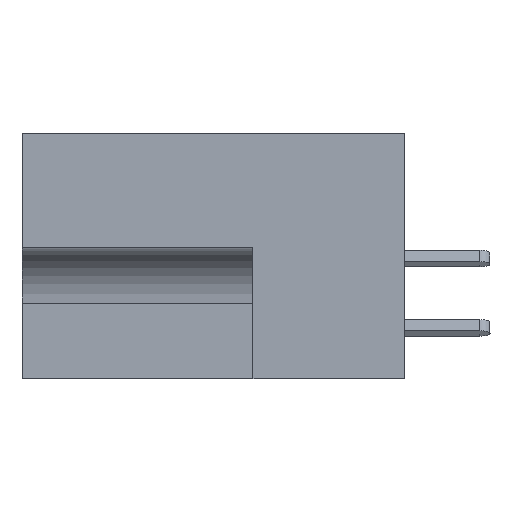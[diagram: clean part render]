
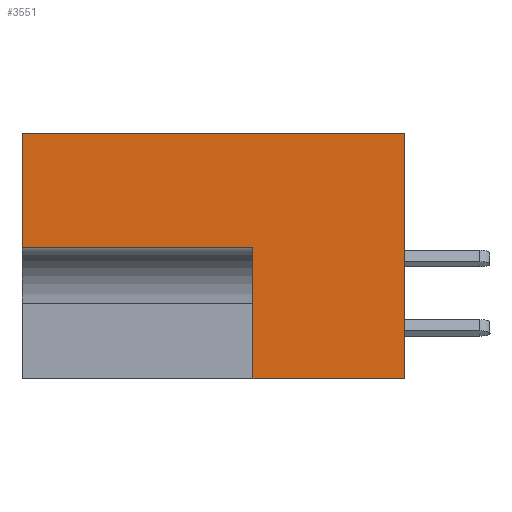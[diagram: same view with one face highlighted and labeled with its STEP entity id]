
A CAD part, left-side view. The second image highlights one B-rep face of the part: STEP entity #3551.
In plain terms, the highlighted planar face has unit normal (-1, 0, 0).
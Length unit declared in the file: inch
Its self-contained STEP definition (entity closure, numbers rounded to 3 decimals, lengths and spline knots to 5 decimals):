
#204 = VERTEX_POINT ( 'NONE', #14856 ) ;
#219 = LINE ( 'NONE', #20313, #17202 ) ;
#373 = DIRECTION ( 'NONE',  ( 0., -1., 0. ) ) ;
#418 = LINE ( 'NONE', #9601, #9098 ) ;
#633 = DIRECTION ( 'NONE',  ( 0., 0., 1. ) ) ;
#1474 = EDGE_CURVE ( 'NONE', #8236, #1812, #13132, .T. ) ;
#1812 = VERTEX_POINT ( 'NONE', #20797 ) ;
#2389 = VECTOR ( 'NONE', #18002, 39.37008 ) ;
#2929 = CARTESIAN_POINT ( 'NONE',  ( 0., 0.328, -0.531 ) ) ;
#3551 = ADVANCED_FACE ( 'NONE', ( #16858 ), #7115, .F. ) ;
#4475 = LINE ( 'NONE', #2929, #2389 ) ;
#4581 = EDGE_CURVE ( 'NONE', #20602, #10920, #5206, .T. ) ;
#5206 = LINE ( 'NONE', #12633, #23700 ) ;
#7115 = PLANE ( 'NONE',  #20609 ) ;
#7203 = CARTESIAN_POINT ( 'NONE',  ( 0., 0.453, 0. ) ) ;
#7913 = CARTESIAN_POINT ( 'NONE',  ( 0., 0.828, 0. ) ) ;
#8236 = VERTEX_POINT ( 'NONE', #7913 ) ;
#8436 = CARTESIAN_POINT ( 'NONE',  ( 0., 0.328, -0.531 ) ) ;
#8957 = DIRECTION ( 'NONE',  ( 0., -1., 0. ) ) ;
#9098 = VECTOR ( 'NONE', #22949, 39.37008 ) ;
#9601 = CARTESIAN_POINT ( 'NONE',  ( 0., 0.328, -0.248 ) ) ;
#9984 = ORIENTED_EDGE ( 'NONE', *, *, #19945, .F. ) ;
#10920 = VERTEX_POINT ( 'NONE', #23550 ) ;
#11828 = CARTESIAN_POINT ( 'NONE',  ( 0., 0.453, 0. ) ) ;
#12633 = CARTESIAN_POINT ( 'NONE',  ( 0., 0.453, -0.531 ) ) ;
#13132 = LINE ( 'NONE', #11828, #21458 ) ;
#13615 = EDGE_LOOP ( 'NONE', ( #21843, #13943, #9984, #23744, #18400, #23489 ) ) ;
#13943 = ORIENTED_EDGE ( 'NONE', *, *, #22816, .F. ) ;
#14712 = DIRECTION ( 'NONE',  ( 0., 0., 1. ) ) ;
#14856 = CARTESIAN_POINT ( 'NONE',  ( 0., 0.328, -0.248 ) ) ;
#16858 = FACE_OUTER_BOUND ( 'NONE', #13615, .T. ) ;
#17202 = VECTOR ( 'NONE', #14712, 39.37008 ) ;
#18002 = DIRECTION ( 'NONE',  ( 0., 0., 1. ) ) ;
#18400 = ORIENTED_EDGE ( 'NONE', *, *, #21176, .T. ) ;
#18692 = DIRECTION ( 'NONE',  ( 1., 0., 0. ) ) ;
#18996 = EDGE_CURVE ( 'NONE', #23163, #8236, #23102, .T. ) ;
#19629 = CARTESIAN_POINT ( 'NONE',  ( 0., 0.828, 0. ) ) ;
#19945 = EDGE_CURVE ( 'NONE', #20602, #204, #4475, .T. ) ;
#20313 = CARTESIAN_POINT ( 'NONE',  ( 0., 0., 0. ) ) ;
#20602 = VERTEX_POINT ( 'NONE', #8436 ) ;
#20609 = AXIS2_PLACEMENT_3D ( 'NONE', #7203, #18692, #20622 ) ;
#20622 = DIRECTION ( 'NONE',  ( 0., 0., -1. ) ) ;
#20797 = CARTESIAN_POINT ( 'NONE',  ( 0., 0., 0. ) ) ;
#21176 = EDGE_CURVE ( 'NONE', #10920, #1812, #219, .T. ) ;
#21458 = VECTOR ( 'NONE', #373, 39.37008 ) ;
#21843 = ORIENTED_EDGE ( 'NONE', *, *, #18996, .F. ) ;
#22487 = VECTOR ( 'NONE', #633, 39.37008 ) ;
#22816 = EDGE_CURVE ( 'NONE', #204, #23163, #418, .T. ) ;
#22949 = DIRECTION ( 'NONE',  ( 0., 1., 0. ) ) ;
#23102 = LINE ( 'NONE', #19629, #22487 ) ;
#23163 = VERTEX_POINT ( 'NONE', #24621 ) ;
#23489 = ORIENTED_EDGE ( 'NONE', *, *, #1474, .F. ) ;
#23550 = CARTESIAN_POINT ( 'NONE',  ( 0., 0., -0.531 ) ) ;
#23700 = VECTOR ( 'NONE', #8957, 39.37008 ) ;
#23744 = ORIENTED_EDGE ( 'NONE', *, *, #4581, .T. ) ;
#24621 = CARTESIAN_POINT ( 'NONE',  ( 0., 0.828, -0.248 ) ) ;
